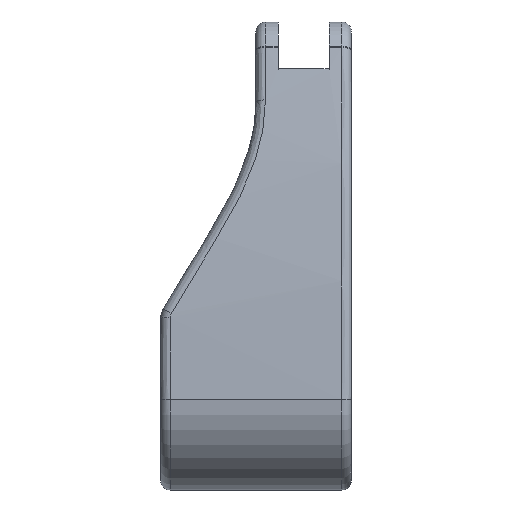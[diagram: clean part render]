
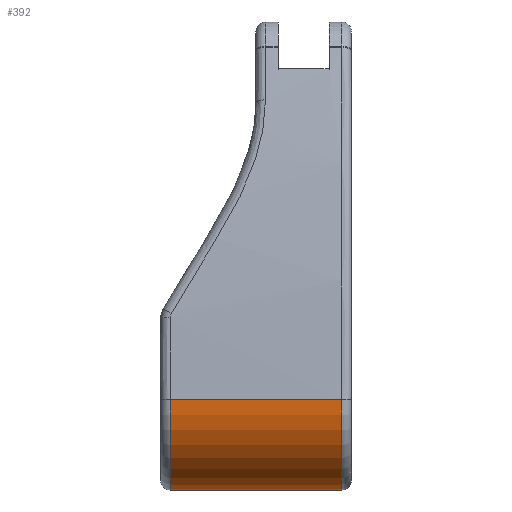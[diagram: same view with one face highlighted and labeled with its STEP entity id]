
A CAD part, left-side view. The second image highlights one B-rep face of the part: STEP entity #392.
In plain terms, the highlighted cylindrical face has radius 28.5 mm (diameter 57 mm), a partial arc.
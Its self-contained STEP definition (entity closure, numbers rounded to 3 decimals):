
#123 = CARTESIAN_POINT ( 'NONE',  ( -28.5, 3., 3.8 ) ) ;
#160 = LINE ( 'NONE', #1455, #1668 ) ;
#296 = EDGE_CURVE ( 'NONE', #472, #2624, #1227, .T. ) ;
#299 = DIRECTION ( 'NONE',  ( 0., -1., 0. ) ) ;
#345 = CARTESIAN_POINT ( 'NONE',  ( 0., 3., -24.7 ) ) ;
#392 = ADVANCED_FACE ( 'NONE', ( #1095 ), #2376, .T. ) ;
#449 = CARTESIAN_POINT ( 'NONE',  ( 0., 60., 3.8 ) ) ;
#472 = VERTEX_POINT ( 'NONE', #4016 ) ;
#597 = CARTESIAN_POINT ( 'NONE',  ( 0., 60., -24.7 ) ) ;
#660 = CIRCLE ( 'NONE', #2404, 28.5 ) ;
#1095 = FACE_OUTER_BOUND ( 'NONE', #2060, .T. ) ;
#1199 = AXIS2_PLACEMENT_3D ( 'NONE', #449, #2394, #1738 ) ;
#1227 = LINE ( 'NONE', #597, #3228 ) ;
#1254 = EDGE_CURVE ( 'NONE', #2624, #4165, #660, .T. ) ;
#1378 = DIRECTION ( 'NONE',  ( 0., 0., 1. ) ) ;
#1455 = CARTESIAN_POINT ( 'NONE',  ( -28.5, 60., 3.8 ) ) ;
#1668 = VECTOR ( 'NONE', #2742, 1000. ) ;
#1674 = EDGE_CURVE ( 'NONE', #1845, #472, #3576, .T. ) ;
#1693 = DIRECTION ( 'NONE',  ( 0., 1., 0. ) ) ;
#1738 = DIRECTION ( 'NONE',  ( 0., 0., -1. ) ) ;
#1845 = VERTEX_POINT ( 'NONE', #3219 ) ;
#2060 = EDGE_LOOP ( 'NONE', ( #3787, #2792, #3986, #2082 ) ) ;
#2082 = ORIENTED_EDGE ( 'NONE', *, *, #3765, .F. ) ;
#2376 = CYLINDRICAL_SURFACE ( 'NONE', #1199, 28.5 ) ;
#2394 = DIRECTION ( 'NONE',  ( 0., -1., 0. ) ) ;
#2404 = AXIS2_PLACEMENT_3D ( 'NONE', #3911, #1693, #1378 ) ;
#2624 = VERTEX_POINT ( 'NONE', #345 ) ;
#2742 = DIRECTION ( 'NONE',  ( 0., -1., 0. ) ) ;
#2792 = ORIENTED_EDGE ( 'NONE', *, *, #296, .T. ) ;
#3168 = DIRECTION ( 'NONE',  ( 0., -1., 0. ) ) ;
#3219 = CARTESIAN_POINT ( 'NONE',  ( -28.5, 57., 3.8 ) ) ;
#3228 = VECTOR ( 'NONE', #3168, 1000. ) ;
#3467 = DIRECTION ( 'NONE',  ( 0., 0., 1. ) ) ;
#3576 = CIRCLE ( 'NONE', #4121, 28.5 ) ;
#3765 = EDGE_CURVE ( 'NONE', #1845, #4165, #160, .T. ) ;
#3787 = ORIENTED_EDGE ( 'NONE', *, *, #1674, .T. ) ;
#3911 = CARTESIAN_POINT ( 'NONE',  ( 0., 3., 3.8 ) ) ;
#3986 = ORIENTED_EDGE ( 'NONE', *, *, #1254, .T. ) ;
#4016 = CARTESIAN_POINT ( 'NONE',  ( 0., 57., -24.7 ) ) ;
#4121 = AXIS2_PLACEMENT_3D ( 'NONE', #4124, #299, #3467 ) ;
#4124 = CARTESIAN_POINT ( 'NONE',  ( 0., 57., 3.8 ) ) ;
#4165 = VERTEX_POINT ( 'NONE', #123 ) ;
